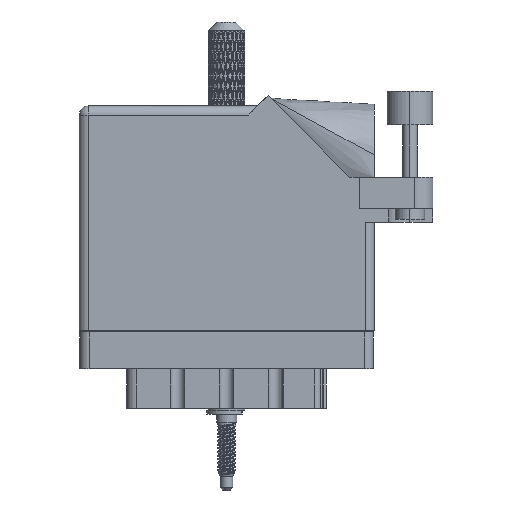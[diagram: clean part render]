
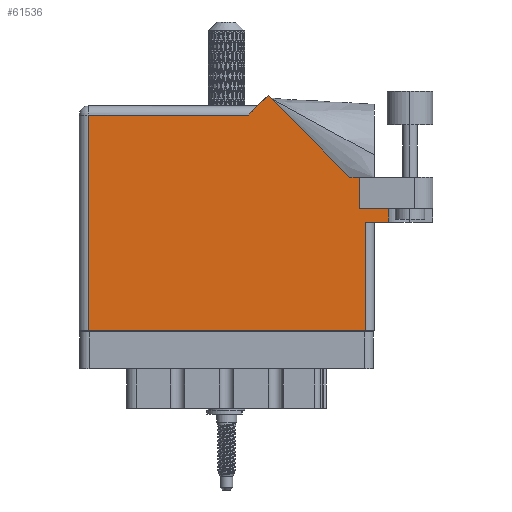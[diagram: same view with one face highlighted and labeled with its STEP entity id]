
A CAD part, front view. The second image highlights one B-rep face of the part: STEP entity #61536.
In plain terms, the highlighted face is planar.
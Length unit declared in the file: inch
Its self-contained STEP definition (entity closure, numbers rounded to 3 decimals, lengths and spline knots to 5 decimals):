
#159 = VERTEX_POINT ( 'NONE', #47486 ) ;
#2588 = CARTESIAN_POINT ( 'NONE',  ( 1.91, 0.831, 0. ) ) ;
#3408 = EDGE_CURVE ( 'NONE', #159, #88610, #40596, .T. ) ;
#4628 = LINE ( 'NONE', #85265, #87652 ) ;
#5785 = CARTESIAN_POINT ( 'NONE',  ( 1.948, 0.737, 0. ) ) ;
#6570 = CARTESIAN_POINT ( 'NONE',  ( 2.01, 0.737, 0. ) ) ;
#8634 = CARTESIAN_POINT ( 'NONE',  ( 0.062, 0., 0. ) ) ;
#11206 = VECTOR ( 'NONE', #43903, 39.37008 ) ;
#12393 = LINE ( 'NONE', #87013, #69408 ) ;
#13174 = EDGE_CURVE ( 'NONE', #101343, #159, #58017, .T. ) ;
#14836 = CARTESIAN_POINT ( 'NONE',  ( 1.84442, 1.044, 0. ) ) ;
#15179 = VERTEX_POINT ( 'NONE', #66311 ) ;
#15485 = DIRECTION ( 'NONE',  ( 0., 1., 0. ) ) ;
#16624 = CARTESIAN_POINT ( 'NONE',  ( 1.91, 0.831, 0. ) ) ;
#19217 = DIRECTION ( 'NONE',  ( -1., 0., 0. ) ) ;
#19804 = VERTEX_POINT ( 'NONE', #26732 ) ;
#20028 = PLANE ( 'NONE',  #32349 ) ;
#20184 = EDGE_CURVE ( 'NONE', #90382, #67614, #22353, .T. ) ;
#21362 = DIRECTION ( 'NONE',  ( 0., -1., 0. ) ) ;
#21461 = EDGE_CURVE ( 'NONE', #73664, #101343, #71473, .T. ) ;
#22353 = LINE ( 'NONE', #58194, #85929 ) ;
#26524 = DIRECTION ( 'NONE',  ( 1., 0., 0. ) ) ;
#26732 = CARTESIAN_POINT ( 'NONE',  ( 2.1115, 0.831, 0. ) ) ;
#30558 = DIRECTION ( 'NONE',  ( -1., 0., 0. ) ) ;
#30871 = ORIENTED_EDGE ( 'NONE', *, *, #61804, .T. ) ;
#31111 = ORIENTED_EDGE ( 'NONE', *, *, #21461, .T. ) ;
#32349 = AXIS2_PLACEMENT_3D ( 'NONE', #54824, #87488, #30558 ) ;
#34677 = EDGE_LOOP ( 'NONE', ( #56610, #102418, #92913, #65431, #67495, #71345, #69549, #106891, #88007, #30871, #31111 ) ) ;
#39626 = CARTESIAN_POINT ( 'NONE',  ( 0., 1.468, 0. ) ) ;
#40596 = LINE ( 'NONE', #5785, #75775 ) ;
#42342 = LINE ( 'NONE', #6570, #44975 ) ;
#43903 = DIRECTION ( 'NONE',  ( 1., 0., 0. ) ) ;
#44975 = VECTOR ( 'NONE', #64571, 39.37008 ) ;
#47486 = CARTESIAN_POINT ( 'NONE',  ( 1.948, 0., 0. ) ) ;
#50711 = DIRECTION ( 'NONE',  ( 0., 1., 0. ) ) ;
#53356 = EDGE_CURVE ( 'NONE', #80502, #90382, #4628, .T. ) ;
#53489 = EDGE_CURVE ( 'NONE', #19804, #75263, #12393, .T. ) ;
#54140 = VECTOR ( 'NONE', #26524, 39.37008 ) ;
#54776 = CARTESIAN_POINT ( 'NONE',  ( 2.1115, 0.737, 0. ) ) ;
#54824 = CARTESIAN_POINT ( 'NONE',  ( 0., 1.53, 0. ) ) ;
#54936 = FACE_OUTER_BOUND ( 'NONE', #34677, .T. ) ;
#56610 = ORIENTED_EDGE ( 'NONE', *, *, #13174, .T. ) ;
#58017 = LINE ( 'NONE', #76947, #54140 ) ;
#58194 = CARTESIAN_POINT ( 'NONE',  ( 1.84442, 1.044, 0. ) ) ;
#59247 = VERTEX_POINT ( 'NONE', #74286 ) ;
#60052 = VECTOR ( 'NONE', #65336, 39.37008 ) ;
#61536 = ADVANCED_FACE ( 'NONE', ( #54936 ), #20028, .F. ) ;
#61804 = EDGE_CURVE ( 'NONE', #15179, #73664, #83493, .T. ) ;
#64571 = DIRECTION ( 'NONE',  ( 1., 0., 0. ) ) ;
#65336 = DIRECTION ( 'NONE',  ( -1., 0., 0. ) ) ;
#65431 = ORIENTED_EDGE ( 'NONE', *, *, #53489, .F. ) ;
#66311 = CARTESIAN_POINT ( 'NONE',  ( 1.155, 1.468, 0. ) ) ;
#67495 = ORIENTED_EDGE ( 'NONE', *, *, #96872, .F. ) ;
#67614 = VERTEX_POINT ( 'NONE', #91743 ) ;
#68685 = DIRECTION ( 'NONE',  ( -0.707, 0.707, 0. ) ) ;
#69408 = VECTOR ( 'NONE', #21362, 39.37008 ) ;
#69549 = ORIENTED_EDGE ( 'NONE', *, *, #53356, .T. ) ;
#70090 = VECTOR ( 'NONE', #78998, 39.37008 ) ;
#71345 = ORIENTED_EDGE ( 'NONE', *, *, #92740, .T. ) ;
#71473 = LINE ( 'NONE', #104975, #70090 ) ;
#71844 = LINE ( 'NONE', #82044, #80920 ) ;
#73322 = CARTESIAN_POINT ( 'NONE',  ( 0.062, 1.468, 0. ) ) ;
#73664 = VERTEX_POINT ( 'NONE', #73322 ) ;
#74286 = CARTESIAN_POINT ( 'NONE',  ( 1.91, 0.831, 0. ) ) ;
#75263 = VERTEX_POINT ( 'NONE', #54776 ) ;
#75306 = EDGE_CURVE ( 'NONE', #88610, #75263, #42342, .T. ) ;
#75775 = VECTOR ( 'NONE', #15485, 39.37008 ) ;
#76947 = CARTESIAN_POINT ( 'NONE',  ( 0., 0., 0. ) ) ;
#78998 = DIRECTION ( 'NONE',  ( 0., -1., 0. ) ) ;
#79654 = EDGE_CURVE ( 'NONE', #67614, #15179, #71844, .T. ) ;
#80502 = VERTEX_POINT ( 'NONE', #83819 ) ;
#80920 = VECTOR ( 'NONE', #106573, 39.37008 ) ;
#82044 = CARTESIAN_POINT ( 'NONE',  ( 1.217, 1.53, 0. ) ) ;
#83493 = LINE ( 'NONE', #39626, #60052 ) ;
#83819 = CARTESIAN_POINT ( 'NONE',  ( 1.91, 1.044, 0. ) ) ;
#85260 = LINE ( 'NONE', #2588, #11206 ) ;
#85265 = CARTESIAN_POINT ( 'NONE',  ( 2.41, 1.044, 0. ) ) ;
#85929 = VECTOR ( 'NONE', #68685, 39.37008 ) ;
#87013 = CARTESIAN_POINT ( 'NONE',  ( 2.1115, 1.16177, 0. ) ) ;
#87488 = DIRECTION ( 'NONE',  ( 0., 0., -1. ) ) ;
#87652 = VECTOR ( 'NONE', #19217, 39.37008 ) ;
#88007 = ORIENTED_EDGE ( 'NONE', *, *, #79654, .T. ) ;
#88610 = VERTEX_POINT ( 'NONE', #102369 ) ;
#90382 = VERTEX_POINT ( 'NONE', #14836 ) ;
#91743 = CARTESIAN_POINT ( 'NONE',  ( 1.28771, 1.60071, 0. ) ) ;
#92027 = VECTOR ( 'NONE', #50711, 39.37008 ) ;
#92740 = EDGE_CURVE ( 'NONE', #59247, #80502, #95968, .T. ) ;
#92913 = ORIENTED_EDGE ( 'NONE', *, *, #75306, .T. ) ;
#95968 = LINE ( 'NONE', #16624, #92027 ) ;
#96872 = EDGE_CURVE ( 'NONE', #59247, #19804, #85260, .T. ) ;
#101343 = VERTEX_POINT ( 'NONE', #8634 ) ;
#102369 = CARTESIAN_POINT ( 'NONE',  ( 1.948, 0.737, 0. ) ) ;
#102418 = ORIENTED_EDGE ( 'NONE', *, *, #3408, .T. ) ;
#104975 = CARTESIAN_POINT ( 'NONE',  ( 0.062, 0., 0. ) ) ;
#106573 = DIRECTION ( 'NONE',  ( -0.707, -0.707, 0. ) ) ;
#106891 = ORIENTED_EDGE ( 'NONE', *, *, #20184, .T. ) ;
